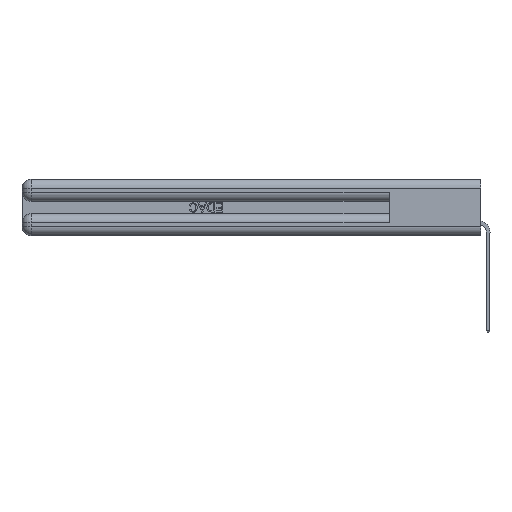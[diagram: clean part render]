
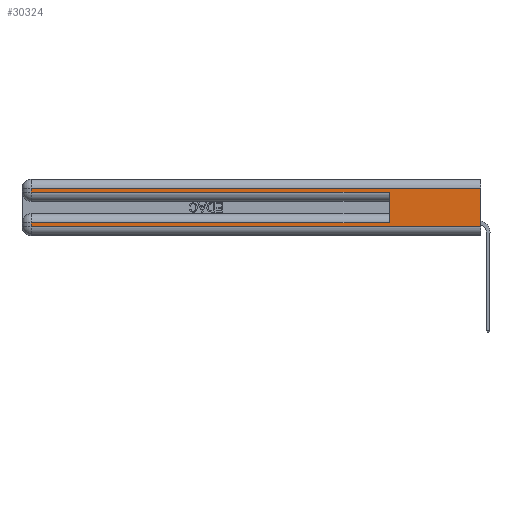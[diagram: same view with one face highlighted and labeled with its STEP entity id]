
A CAD part, left-side view. The second image highlights one B-rep face of the part: STEP entity #30324.
In plain terms, the highlighted planar face has unit normal (-1, 0, 0).
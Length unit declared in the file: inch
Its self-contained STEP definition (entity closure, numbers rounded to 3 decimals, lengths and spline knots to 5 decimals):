
#139 = VERTEX_POINT ( 'NONE', #21537 ) ;
#223 = VECTOR ( 'NONE', #36014, 39.37008 ) ;
#236 = ORIENTED_EDGE ( 'NONE', *, *, #29057, .T. ) ;
#1437 = VERTEX_POINT ( 'NONE', #4742 ) ;
#1890 = LINE ( 'NONE', #3846, #23929 ) ;
#3818 = CARTESIAN_POINT ( 'NONE',  ( 0., 0., 0.285 ) ) ;
#3846 = CARTESIAN_POINT ( 'NONE',  ( 0., 2.94, 0.37 ) ) ;
#4348 = LINE ( 'NONE', #35883, #223 ) ;
#4742 = CARTESIAN_POINT ( 'NONE',  ( 0., 2.94, 0.085 ) ) ;
#4858 = EDGE_CURVE ( 'NONE', #1437, #139, #21296, .T. ) ;
#5850 = LINE ( 'NONE', #29536, #30279 ) ;
#5926 = EDGE_CURVE ( 'NONE', #23767, #29313, #1890, .T. ) ;
#6380 = VECTOR ( 'NONE', #15664, 39.37008 ) ;
#6564 = AXIS2_PLACEMENT_3D ( 'NONE', #28956, #11668, #34796 ) ;
#6858 = DIRECTION ( 'NONE',  ( 0., 0., -1. ) ) ;
#7781 = CARTESIAN_POINT ( 'NONE',  ( 0., 2.94, 0.31 ) ) ;
#8732 = PLANE ( 'NONE',  #6564 ) ;
#9093 = EDGE_CURVE ( 'NONE', #17544, #23767, #4348, .T. ) ;
#11668 = DIRECTION ( 'NONE',  ( 1., 0., 0. ) ) ;
#12304 = ORIENTED_EDGE ( 'NONE', *, *, #4858, .T. ) ;
#14138 = LINE ( 'NONE', #3818, #26341 ) ;
#15368 = DIRECTION ( 'NONE',  ( 0., -1., 0. ) ) ;
#15504 = ORIENTED_EDGE ( 'NONE', *, *, #32744, .T. ) ;
#15664 = DIRECTION ( 'NONE',  ( 0., 0., -1. ) ) ;
#15880 = LINE ( 'NONE', #33414, #6380 ) ;
#16411 = ORIENTED_EDGE ( 'NONE', *, *, #5926, .T. ) ;
#16818 = ORIENTED_EDGE ( 'NONE', *, *, #24595, .F. ) ;
#17008 = FACE_OUTER_BOUND ( 'NONE', #24102, .T. ) ;
#17544 = VERTEX_POINT ( 'NONE', #25191 ) ;
#18446 = VERTEX_POINT ( 'NONE', #20997 ) ;
#18542 = LINE ( 'NONE', #27736, #19459 ) ;
#19459 = VECTOR ( 'NONE', #24568, 39.37008 ) ;
#20664 = CARTESIAN_POINT ( 'NONE',  ( 0., 2.94, 0.285 ) ) ;
#20774 = VECTOR ( 'NONE', #31885, 39.37008 ) ;
#20997 = CARTESIAN_POINT ( 'NONE',  ( 0., 0.6, 0.285 ) ) ;
#21296 = LINE ( 'NONE', #30174, #33605 ) ;
#21537 = CARTESIAN_POINT ( 'NONE',  ( 0., 2.94, 0.06 ) ) ;
#21905 = CARTESIAN_POINT ( 'NONE',  ( 0., 0.6, 0.085 ) ) ;
#21908 = EDGE_CURVE ( 'NONE', #25120, #1437, #34402, .T. ) ;
#23767 = VERTEX_POINT ( 'NONE', #7781 ) ;
#23928 = EDGE_CURVE ( 'NONE', #17544, #31382, #15880, .T. ) ;
#23929 = VECTOR ( 'NONE', #6858, 39.37008 ) ;
#24102 = EDGE_LOOP ( 'NONE', ( #30516, #29247, #16411, #15504, #16818, #27384, #12304, #236 ) ) ;
#24568 = DIRECTION ( 'NONE',  ( 0., 0., 1. ) ) ;
#24595 = EDGE_CURVE ( 'NONE', #25120, #18446, #18542, .T. ) ;
#25120 = VERTEX_POINT ( 'NONE', #21905 ) ;
#25191 = CARTESIAN_POINT ( 'NONE',  ( 0., 0., 0.31 ) ) ;
#26341 = VECTOR ( 'NONE', #15368, 39.37008 ) ;
#26731 = DIRECTION ( 'NONE',  ( 0., -1., 0. ) ) ;
#27384 = ORIENTED_EDGE ( 'NONE', *, *, #21908, .T. ) ;
#27736 = CARTESIAN_POINT ( 'NONE',  ( 0., 0.6, 0.145 ) ) ;
#28147 = CARTESIAN_POINT ( 'NONE',  ( 0., 0., 0.06 ) ) ;
#28956 = CARTESIAN_POINT ( 'NONE',  ( 0., 0., 0.37 ) ) ;
#29057 = EDGE_CURVE ( 'NONE', #139, #31382, #5850, .T. ) ;
#29247 = ORIENTED_EDGE ( 'NONE', *, *, #9093, .T. ) ;
#29313 = VERTEX_POINT ( 'NONE', #20664 ) ;
#29536 = CARTESIAN_POINT ( 'NONE',  ( 0., 0., 0.06 ) ) ;
#30174 = CARTESIAN_POINT ( 'NONE',  ( 0., 2.94, 0.37 ) ) ;
#30279 = VECTOR ( 'NONE', #26731, 39.37008 ) ;
#30324 = ADVANCED_FACE ( 'NONE', ( #17008 ), #8732, .F. ) ;
#30516 = ORIENTED_EDGE ( 'NONE', *, *, #23928, .F. ) ;
#31382 = VERTEX_POINT ( 'NONE', #28147 ) ;
#31885 = DIRECTION ( 'NONE',  ( 0., 1., 0. ) ) ;
#32744 = EDGE_CURVE ( 'NONE', #29313, #18446, #14138, .T. ) ;
#33414 = CARTESIAN_POINT ( 'NONE',  ( 0., 0., 0.37 ) ) ;
#33605 = VECTOR ( 'NONE', #36813, 39.37008 ) ;
#34402 = LINE ( 'NONE', #34899, #20774 ) ;
#34796 = DIRECTION ( 'NONE',  ( 0., 0., -1. ) ) ;
#34899 = CARTESIAN_POINT ( 'NONE',  ( 0., 0., 0.085 ) ) ;
#35883 = CARTESIAN_POINT ( 'NONE',  ( 0., 0., 0.31 ) ) ;
#36014 = DIRECTION ( 'NONE',  ( 0., 1., 0. ) ) ;
#36813 = DIRECTION ( 'NONE',  ( 0., 0., -1. ) ) ;
